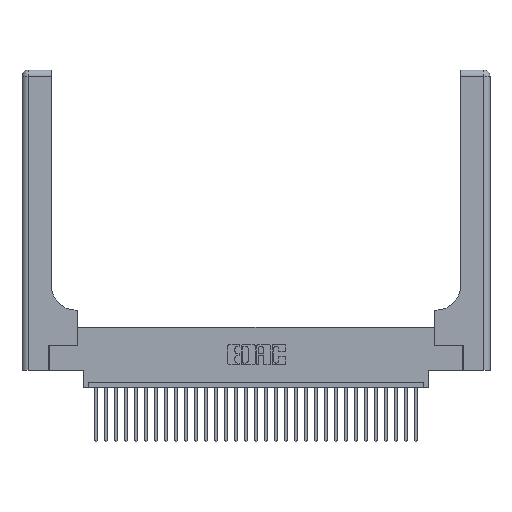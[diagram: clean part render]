
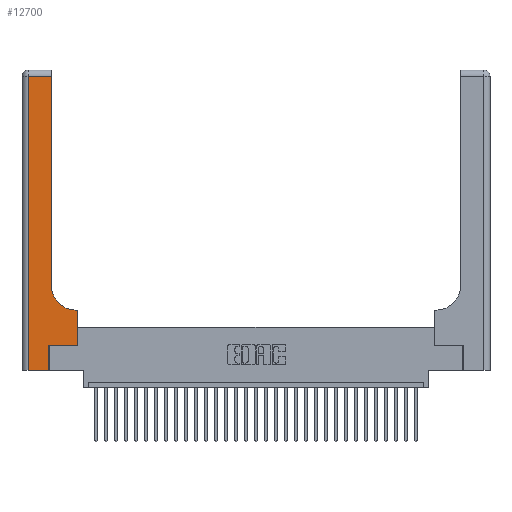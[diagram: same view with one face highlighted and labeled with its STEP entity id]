
A CAD part, top view. The second image highlights one B-rep face of the part: STEP entity #12700.
In plain terms, the highlighted planar face has unit normal (0, 0, 1).
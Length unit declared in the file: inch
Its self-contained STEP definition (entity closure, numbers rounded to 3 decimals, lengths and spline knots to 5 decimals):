
#272 = CARTESIAN_POINT ( 'NONE',  ( 0.06, 2.94, 0.37 ) ) ;
#290 = VERTEX_POINT ( 'NONE', #9958 ) ;
#328 = AXIS2_PLACEMENT_3D ( 'NONE', #7938, #25098, #11309 ) ;
#1197 = ORIENTED_EDGE ( 'NONE', *, *, #4687, .T. ) ;
#2002 = CARTESIAN_POINT ( 'NONE',  ( 0.2915, 2.94, 0.37 ) ) ;
#2798 = DIRECTION ( 'NONE',  ( 0., 1., 0. ) ) ;
#2880 = VERTEX_POINT ( 'NONE', #3693 ) ;
#3598 = CARTESIAN_POINT ( 'NONE',  ( 0.5415, 0.85, 0.37 ) ) ;
#3690 = CARTESIAN_POINT ( 'NONE',  ( 0.269, 0.25, 0.37 ) ) ;
#3693 = CARTESIAN_POINT ( 'NONE',  ( 0.5585, 0.25, 0.37 ) ) ;
#4687 = EDGE_CURVE ( 'NONE', #11473, #290, #23286, .T. ) ;
#4938 = LINE ( 'NONE', #10732, #13688 ) ;
#4951 = CARTESIAN_POINT ( 'NONE',  ( 0.5585, 0.6, 0.37 ) ) ;
#5183 = ORIENTED_EDGE ( 'NONE', *, *, #11607, .T. ) ;
#5349 = LINE ( 'NONE', #30207, #19393 ) ;
#5611 = EDGE_CURVE ( 'NONE', #12262, #24701, #17473, .T. ) ;
#5660 = VERTEX_POINT ( 'NONE', #6240 ) ;
#6240 = CARTESIAN_POINT ( 'NONE',  ( 0.269, 0., 0.37 ) ) ;
#6251 = FACE_OUTER_BOUND ( 'NONE', #28867, .T. ) ;
#6611 = EDGE_CURVE ( 'NONE', #2880, #20553, #21187, .T. ) ;
#7513 = VECTOR ( 'NONE', #2798, 39.37008 ) ;
#7938 = CARTESIAN_POINT ( 'NONE',  ( 0., 3., 0.37 ) ) ;
#7999 = DIRECTION ( 'NONE',  ( -1., 0., 0. ) ) ;
#9091 = ORIENTED_EDGE ( 'NONE', *, *, #5611, .T. ) ;
#9835 = CARTESIAN_POINT ( 'NONE',  ( 0., 0., 0.37 ) ) ;
#9868 = CARTESIAN_POINT ( 'NONE',  ( 0.06, 3., 0.37 ) ) ;
#9958 = CARTESIAN_POINT ( 'NONE',  ( 0.2915, 0.85, 0.37 ) ) ;
#10585 = DIRECTION ( 'NONE',  ( 0., 0., -1. ) ) ;
#10732 = CARTESIAN_POINT ( 'NONE',  ( 0.2915, 0.6, 0.37 ) ) ;
#11015 = VECTOR ( 'NONE', #12098, 39.37008 ) ;
#11017 = VERTEX_POINT ( 'NONE', #3690 ) ;
#11309 = DIRECTION ( 'NONE',  ( -1., 0., 0. ) ) ;
#11473 = VERTEX_POINT ( 'NONE', #17443 ) ;
#11607 = EDGE_CURVE ( 'NONE', #20553, #11473, #4938, .T. ) ;
#12098 = DIRECTION ( 'NONE',  ( 0., -1., 0. ) ) ;
#12262 = VERTEX_POINT ( 'NONE', #272 ) ;
#12396 = LINE ( 'NONE', #9835, #30925 ) ;
#12700 = ADVANCED_FACE ( 'NONE', ( #6251 ), #24992, .F. ) ;
#13339 = ORIENTED_EDGE ( 'NONE', *, *, #30406, .T. ) ;
#13531 = ORIENTED_EDGE ( 'NONE', *, *, #6611, .T. ) ;
#13688 = VECTOR ( 'NONE', #7999, 39.37008 ) ;
#13893 = ORIENTED_EDGE ( 'NONE', *, *, #18600, .T. ) ;
#15271 = EDGE_CURVE ( 'NONE', #11017, #2880, #18606, .T. ) ;
#16693 = VECTOR ( 'NONE', #18857, 39.37008 ) ;
#16788 = DIRECTION ( 'NONE',  ( 0., 1., 0. ) ) ;
#17399 = CARTESIAN_POINT ( 'NONE',  ( 0.269, 0., 0.37 ) ) ;
#17443 = CARTESIAN_POINT ( 'NONE',  ( 0.5415, 0.6, 0.37 ) ) ;
#17473 = LINE ( 'NONE', #9868, #11015 ) ;
#17977 = VERTEX_POINT ( 'NONE', #2002 ) ;
#18600 = EDGE_CURVE ( 'NONE', #17977, #12262, #5349, .T. ) ;
#18606 = LINE ( 'NONE', #30143, #16693 ) ;
#18857 = DIRECTION ( 'NONE',  ( 1., 0., 0. ) ) ;
#19215 = LINE ( 'NONE', #17399, #23369 ) ;
#19393 = VECTOR ( 'NONE', #19840, 39.37008 ) ;
#19820 = DIRECTION ( 'NONE',  ( 0., 1., 0. ) ) ;
#19840 = DIRECTION ( 'NONE',  ( -1., 0., 0. ) ) ;
#20088 = ORIENTED_EDGE ( 'NONE', *, *, #15271, .T. ) ;
#20553 = VERTEX_POINT ( 'NONE', #4951 ) ;
#20783 = LINE ( 'NONE', #26855, #7513 ) ;
#21187 = LINE ( 'NONE', #24001, #21936 ) ;
#21651 = EDGE_CURVE ( 'NONE', #24701, #5660, #12396, .T. ) ;
#21766 = AXIS2_PLACEMENT_3D ( 'NONE', #3598, #10585, #27546 ) ;
#21936 = VECTOR ( 'NONE', #16788, 39.37008 ) ;
#22227 = ORIENTED_EDGE ( 'NONE', *, *, #29323, .T. ) ;
#23286 = CIRCLE ( 'NONE', #21766, 0.25 ) ;
#23369 = VECTOR ( 'NONE', #19820, 39.37008 ) ;
#24001 = CARTESIAN_POINT ( 'NONE',  ( 0.5585, 0.25, 0.37 ) ) ;
#24701 = VERTEX_POINT ( 'NONE', #28150 ) ;
#24992 = PLANE ( 'NONE',  #328 ) ;
#25098 = DIRECTION ( 'NONE',  ( 0., 0., -1. ) ) ;
#26855 = CARTESIAN_POINT ( 'NONE',  ( 0.2915, 3., 0.37 ) ) ;
#27546 = DIRECTION ( 'NONE',  ( 1., 0., 0. ) ) ;
#28150 = CARTESIAN_POINT ( 'NONE',  ( 0.06, 0., 0.37 ) ) ;
#28867 = EDGE_LOOP ( 'NONE', ( #22227, #13893, #9091, #31355, #13339, #20088, #13531, #5183, #1197 ) ) ;
#29107 = DIRECTION ( 'NONE',  ( 1., 0., 0. ) ) ;
#29323 = EDGE_CURVE ( 'NONE', #290, #17977, #20783, .T. ) ;
#30143 = CARTESIAN_POINT ( 'NONE',  ( 0.269, 0.25, 0.37 ) ) ;
#30207 = CARTESIAN_POINT ( 'NONE',  ( 0., 2.94, 0.37 ) ) ;
#30406 = EDGE_CURVE ( 'NONE', #5660, #11017, #19215, .T. ) ;
#30925 = VECTOR ( 'NONE', #29107, 39.37008 ) ;
#31355 = ORIENTED_EDGE ( 'NONE', *, *, #21651, .T. ) ;
